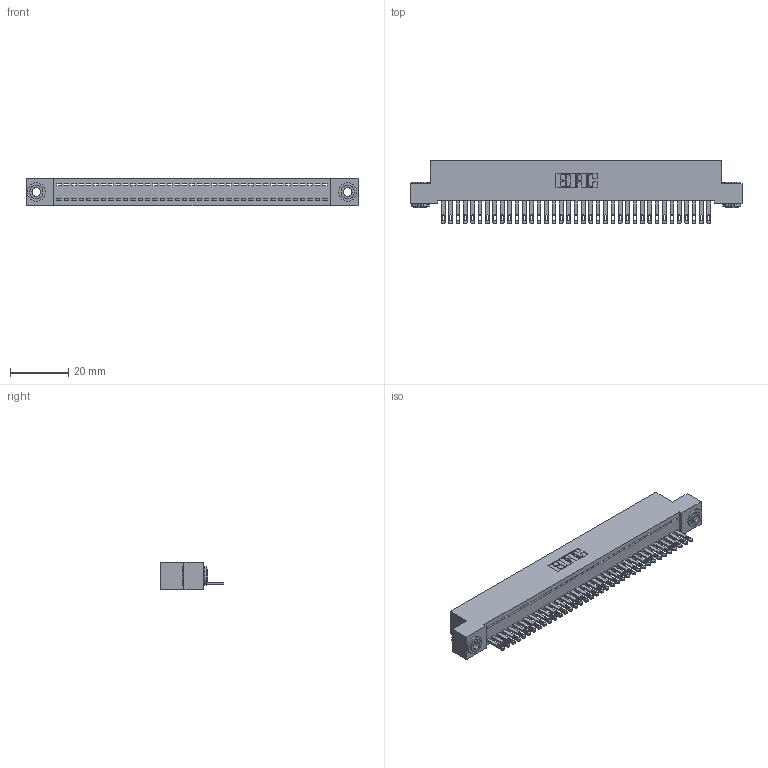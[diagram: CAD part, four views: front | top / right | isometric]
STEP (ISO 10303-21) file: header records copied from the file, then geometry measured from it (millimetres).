
FILE_DESCRIPTION (( 'STEP AP203' ), '1' );
FILE_NAME ('342-037-500-103.STEP', '2018-08-11T21:01:31', ( '' ), ( '' ), 'SwSTEP 2.0', 'SolidWorks 2016', '' );
FILE_SCHEMA (( 'CONFIG_CONTROL_DESIGN' ));
Length unit declared in the file: inch
Products named in the file (4): 342-037-500-103; 342 Part_.156 TH; 345-292-001_345-293-100; 342-250-002_345-250-002-102
Assembly tree (40 placements, depth 2):
  342-037-500-103
    342 Part_.156 TH
    345-292-001_345-293-100  x37
    342-250-002_345-250-002-102  x2
Bounding box: 114.3 x 21.85 x 9.4 mm (x, y, z)
Volume: 10049.1 mm3; surface area: 14962.3 mm2
Topology: 40 solids, 40 shells, 2146 faces, 6591 edges, 4390 vertices
Faces by surface type: plane 1408, cylinder 730, cone 8
Entity records: 23714 total; most frequent: CARTESIAN_POINT 4068, ORIENTED_EDGE 4034, DIRECTION 3477, EDGE_CURVE 2017, LINE 1861, VECTOR 1861, VERTEX_POINT 1342, AXIS2_PLACEMENT_3D 808
